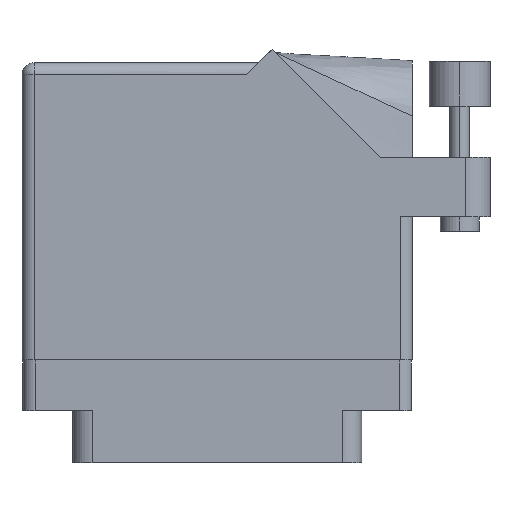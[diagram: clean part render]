
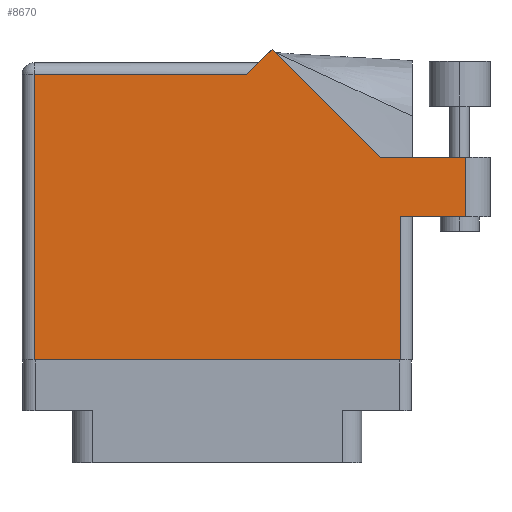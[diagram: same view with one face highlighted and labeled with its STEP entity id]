
A CAD part, front view. The second image highlights one B-rep face of the part: STEP entity #8670.
In plain terms, the highlighted face is planar.
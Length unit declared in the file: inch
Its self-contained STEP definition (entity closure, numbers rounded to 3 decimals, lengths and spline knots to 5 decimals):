
#50 = VECTOR ( 'NONE', #4408, 39.37008 ) ;
#52 = DIRECTION ( 'NONE',  ( -1., 0., 0. ) ) ;
#1085 = CARTESIAN_POINT ( 'NONE',  ( 2.285, 0.737, 0. ) ) ;
#1237 = CARTESIAN_POINT ( 'NONE',  ( 1.948, 0., 0. ) ) ;
#1303 = LINE ( 'NONE', #13099, #31663 ) ;
#1334 = LINE ( 'NONE', #16855, #50 ) ;
#1497 = LINE ( 'NONE', #25174, #14118 ) ;
#2331 = ORIENTED_EDGE ( 'NONE', *, *, #34866, .T. ) ;
#3221 = DIRECTION ( 'NONE',  ( 1., 0., 0. ) ) ;
#3830 = FACE_OUTER_BOUND ( 'NONE', #25640, .T. ) ;
#4183 = CARTESIAN_POINT ( 'NONE',  ( 0.062, 1.468, 0. ) ) ;
#4357 = LINE ( 'NONE', #18269, #19895 ) ;
#4408 = DIRECTION ( 'NONE',  ( 0., 1., 0. ) ) ;
#4609 = CARTESIAN_POINT ( 'NONE',  ( 1.948, 0.737, 0. ) ) ;
#4710 = EDGE_CURVE ( 'NONE', #17023, #10153, #12922, .T. ) ;
#4998 = CARTESIAN_POINT ( 'NONE',  ( 1.155, 1.468, 0. ) ) ;
#5367 = PLANE ( 'NONE',  #20380 ) ;
#6921 = VECTOR ( 'NONE', #3221, 39.37008 ) ;
#7344 = CARTESIAN_POINT ( 'NONE',  ( 1.84442, 1.044, 0. ) ) ;
#7801 = DIRECTION ( 'NONE',  ( -0.707, -0.707, 0. ) ) ;
#8670 = ADVANCED_FACE ( 'NONE', ( #3830 ), #5367, .F. ) ;
#9655 = ORIENTED_EDGE ( 'NONE', *, *, #22086, .T. ) ;
#10153 = VERTEX_POINT ( 'NONE', #30373 ) ;
#10253 = CARTESIAN_POINT ( 'NONE',  ( 0.062, 0., 0. ) ) ;
#10258 = EDGE_CURVE ( 'NONE', #14340, #10780, #1497, .T. ) ;
#10780 = VERTEX_POINT ( 'NONE', #10253 ) ;
#12562 = EDGE_CURVE ( 'NONE', #28188, #14340, #28787, .T. ) ;
#12717 = DIRECTION ( 'NONE',  ( -1., 0., 0. ) ) ;
#12922 = LINE ( 'NONE', #17390, #21329 ) ;
#13099 = CARTESIAN_POINT ( 'NONE',  ( 1.217, 1.53, 0. ) ) ;
#13488 = EDGE_CURVE ( 'NONE', #10153, #14209, #32935, .T. ) ;
#13586 = EDGE_CURVE ( 'NONE', #14209, #28188, #1303, .T. ) ;
#13598 = CARTESIAN_POINT ( 'NONE',  ( 2.285, 1.044, 0. ) ) ;
#14118 = VECTOR ( 'NONE', #14650, 39.37008 ) ;
#14209 = VERTEX_POINT ( 'NONE', #21695 ) ;
#14340 = VERTEX_POINT ( 'NONE', #4183 ) ;
#14650 = DIRECTION ( 'NONE',  ( 0., -1., 0. ) ) ;
#14829 = VERTEX_POINT ( 'NONE', #1237 ) ;
#15754 = ORIENTED_EDGE ( 'NONE', *, *, #13488, .T. ) ;
#15882 = ORIENTED_EDGE ( 'NONE', *, *, #10258, .T. ) ;
#16702 = EDGE_CURVE ( 'NONE', #34472, #17023, #31309, .T. ) ;
#16855 = CARTESIAN_POINT ( 'NONE',  ( 1.948, 0.737, 0. ) ) ;
#17023 = VERTEX_POINT ( 'NONE', #17346 ) ;
#17346 = CARTESIAN_POINT ( 'NONE',  ( 2.285, 1.044, 0. ) ) ;
#17390 = CARTESIAN_POINT ( 'NONE',  ( 2.41, 1.044, 0. ) ) ;
#18269 = CARTESIAN_POINT ( 'NONE',  ( 0., 0., 0. ) ) ;
#19895 = VECTOR ( 'NONE', #23286, 39.37008 ) ;
#20380 = AXIS2_PLACEMENT_3D ( 'NONE', #32007, #32130, #52 ) ;
#21090 = VERTEX_POINT ( 'NONE', #4609 ) ;
#21329 = VECTOR ( 'NONE', #12717, 39.37008 ) ;
#21600 = ORIENTED_EDGE ( 'NONE', *, *, #13586, .T. ) ;
#21695 = CARTESIAN_POINT ( 'NONE',  ( 1.28771, 1.60071, 0. ) ) ;
#22069 = DIRECTION ( 'NONE',  ( 0., 1., 0. ) ) ;
#22086 = EDGE_CURVE ( 'NONE', #10780, #14829, #4357, .T. ) ;
#22652 = ORIENTED_EDGE ( 'NONE', *, *, #12562, .T. ) ;
#23286 = DIRECTION ( 'NONE',  ( 1., 0., 0. ) ) ;
#23359 = LINE ( 'NONE', #32290, #6921 ) ;
#24876 = CARTESIAN_POINT ( 'NONE',  ( 0., 1.468, 0. ) ) ;
#25174 = CARTESIAN_POINT ( 'NONE',  ( 0.062, 0., 0. ) ) ;
#25346 = ORIENTED_EDGE ( 'NONE', *, *, #4710, .T. ) ;
#25640 = EDGE_LOOP ( 'NONE', ( #2331, #31858, #25346, #15754, #21600, #22652, #15882, #9655, #34185 ) ) ;
#25775 = VECTOR ( 'NONE', #26191, 39.37008 ) ;
#25838 = VECTOR ( 'NONE', #32990, 39.37008 ) ;
#26191 = DIRECTION ( 'NONE',  ( -0.707, 0.707, 0. ) ) ;
#26653 = VECTOR ( 'NONE', #22069, 39.37008 ) ;
#26748 = EDGE_CURVE ( 'NONE', #14829, #21090, #1334, .T. ) ;
#28188 = VERTEX_POINT ( 'NONE', #4998 ) ;
#28787 = LINE ( 'NONE', #24876, #25838 ) ;
#30373 = CARTESIAN_POINT ( 'NONE',  ( 1.84442, 1.044, 0. ) ) ;
#31309 = LINE ( 'NONE', #13598, #26653 ) ;
#31663 = VECTOR ( 'NONE', #7801, 39.37008 ) ;
#31858 = ORIENTED_EDGE ( 'NONE', *, *, #16702, .T. ) ;
#32007 = CARTESIAN_POINT ( 'NONE',  ( 0., 1.53, 0. ) ) ;
#32130 = DIRECTION ( 'NONE',  ( 0., 0., -1. ) ) ;
#32290 = CARTESIAN_POINT ( 'NONE',  ( 2.01, 0.737, 0. ) ) ;
#32935 = LINE ( 'NONE', #7344, #25775 ) ;
#32990 = DIRECTION ( 'NONE',  ( -1., 0., 0. ) ) ;
#34185 = ORIENTED_EDGE ( 'NONE', *, *, #26748, .T. ) ;
#34472 = VERTEX_POINT ( 'NONE', #1085 ) ;
#34866 = EDGE_CURVE ( 'NONE', #21090, #34472, #23359, .T. ) ;
